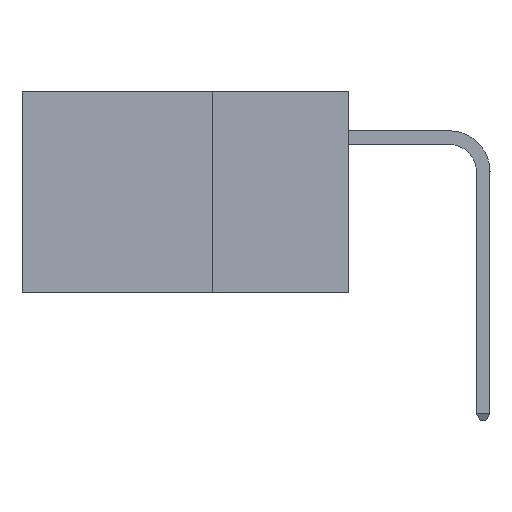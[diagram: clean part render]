
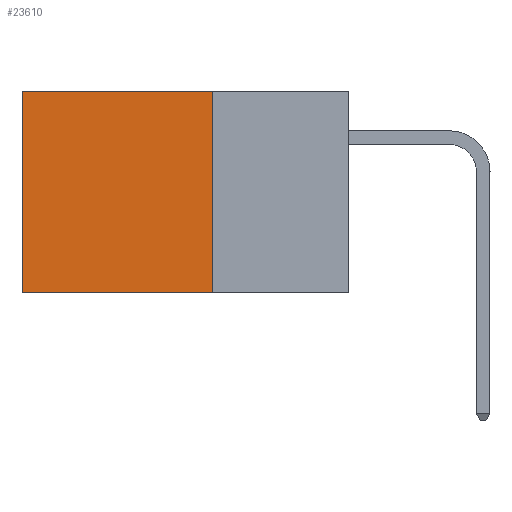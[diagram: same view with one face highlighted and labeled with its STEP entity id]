
A CAD part, left-side view. The second image highlights one B-rep face of the part: STEP entity #23610.
In plain terms, the highlighted planar face has unit normal (-1, 0, 0).
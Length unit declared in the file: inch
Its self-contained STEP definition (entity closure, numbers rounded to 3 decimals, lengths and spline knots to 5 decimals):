
#2420 = CARTESIAN_POINT ( 'NONE',  ( 0.2875, 0.6, 0. ) ) ;
#3205 = VECTOR ( 'NONE', #26060, 39.37008 ) ;
#3567 = CARTESIAN_POINT ( 'NONE',  ( 0.2875, 0.25, -0.37 ) ) ;
#5649 = EDGE_CURVE ( 'NONE', #25913, #31178, #47099, .T. ) ;
#7045 = VECTOR ( 'NONE', #23672, 39.37008 ) ;
#8085 = ORIENTED_EDGE ( 'NONE', *, *, #5649, .F. ) ;
#9780 = CARTESIAN_POINT ( 'NONE',  ( 0.2875, 0.6, -0.37 ) ) ;
#14245 = CARTESIAN_POINT ( 'NONE',  ( 0.2875, 0.25, 0. ) ) ;
#14931 = ORIENTED_EDGE ( 'NONE', *, *, #16898, .F. ) ;
#16546 = CARTESIAN_POINT ( 'NONE',  ( 0.2875, 0.25, 0. ) ) ;
#16898 = EDGE_CURVE ( 'NONE', #35136, #25913, #44822, .T. ) ;
#17568 = CARTESIAN_POINT ( 'NONE',  ( 0.2875, 0.6, 0. ) ) ;
#18902 = ORIENTED_EDGE ( 'NONE', *, *, #31060, .T. ) ;
#18917 = EDGE_CURVE ( 'NONE', #44805, #31178, #23027, .T. ) ;
#21062 = EDGE_LOOP ( 'NONE', ( #27353, #8085, #14931, #18902 ) ) ;
#21069 = CARTESIAN_POINT ( 'NONE',  ( 0.2875, 0.25, 0. ) ) ;
#23027 = LINE ( 'NONE', #2420, #7045 ) ;
#23610 = ADVANCED_FACE ( 'NONE', ( #45294 ), #32340, .F. ) ;
#23672 = DIRECTION ( 'NONE',  ( 0., 0., -1. ) ) ;
#24970 = VECTOR ( 'NONE', #34152, 39.37008 ) ;
#25165 = LINE ( 'NONE', #16546, #38794 ) ;
#25913 = VERTEX_POINT ( 'NONE', #3567 ) ;
#26060 = DIRECTION ( 'NONE',  ( 0., 0., -1. ) ) ;
#27353 = ORIENTED_EDGE ( 'NONE', *, *, #18917, .T. ) ;
#29096 = AXIS2_PLACEMENT_3D ( 'NONE', #21069, #32023, #43322 ) ;
#31060 = EDGE_CURVE ( 'NONE', #35136, #44805, #25165, .T. ) ;
#31178 = VERTEX_POINT ( 'NONE', #9780 ) ;
#32023 = DIRECTION ( 'NONE',  ( 1., 0., 0. ) ) ;
#32340 = PLANE ( 'NONE',  #29096 ) ;
#34152 = DIRECTION ( 'NONE',  ( 0., 1., 0. ) ) ;
#35136 = VERTEX_POINT ( 'NONE', #14245 ) ;
#37518 = CARTESIAN_POINT ( 'NONE',  ( 0.2875, 0.25, -0.37 ) ) ;
#38319 = DIRECTION ( 'NONE',  ( 0., 1., 0. ) ) ;
#38794 = VECTOR ( 'NONE', #38319, 39.37008 ) ;
#43322 = DIRECTION ( 'NONE',  ( 0., 0., -1. ) ) ;
#44794 = CARTESIAN_POINT ( 'NONE',  ( 0.2875, 0.25, 0. ) ) ;
#44805 = VERTEX_POINT ( 'NONE', #17568 ) ;
#44822 = LINE ( 'NONE', #44794, #3205 ) ;
#45294 = FACE_OUTER_BOUND ( 'NONE', #21062, .T. ) ;
#47099 = LINE ( 'NONE', #37518, #24970 ) ;
